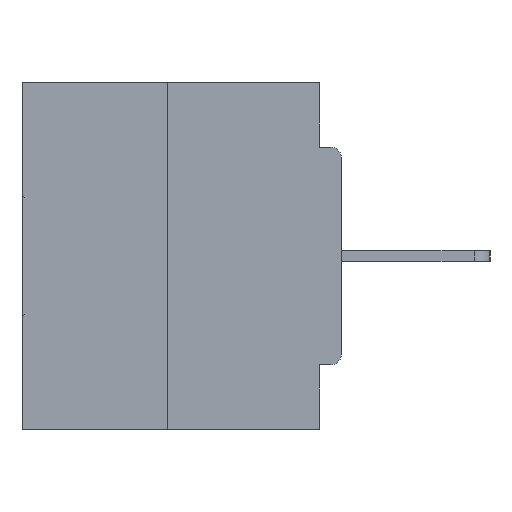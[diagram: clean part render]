
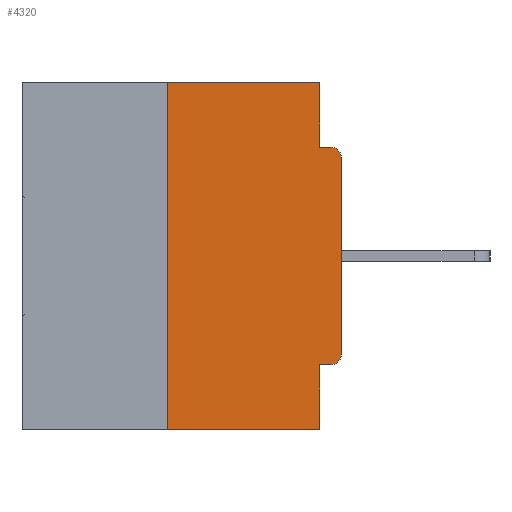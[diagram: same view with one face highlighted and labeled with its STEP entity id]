
A CAD part, left-side view. The second image highlights one B-rep face of the part: STEP entity #4320.
In plain terms, the highlighted planar face has unit normal (-1, 0, 0).
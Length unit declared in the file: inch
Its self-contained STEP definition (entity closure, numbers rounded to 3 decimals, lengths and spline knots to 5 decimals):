
#682 = VERTEX_POINT ( 'NONE', #20227 ) ;
#1584 = LINE ( 'NONE', #30720, #3034 ) ;
#2029 = CARTESIAN_POINT ( 'NONE',  ( 0., 0.46, -0.5 ) ) ;
#2824 = DIRECTION ( 'NONE',  ( 0., 0., -1. ) ) ;
#2882 = CARTESIAN_POINT ( 'NONE',  ( 0., 0.015, -0.3915 ) ) ;
#3034 = VECTOR ( 'NONE', #12272, 39.37008 ) ;
#3341 = AXIS2_PLACEMENT_3D ( 'NONE', #2882, #26212, #32212 ) ;
#3431 = FACE_OUTER_BOUND ( 'NONE', #16127, .T. ) ;
#3579 = CARTESIAN_POINT ( 'NONE',  ( 0., 0.031, -0.5 ) ) ;
#3652 = VECTOR ( 'NONE', #10860, 39.37008 ) ;
#4320 = ADVANCED_FACE ( 'NONE', ( #3431 ), #11691, .F. ) ;
#5598 = ORIENTED_EDGE ( 'NONE', *, *, #26268, .F. ) ;
#5643 = LINE ( 'NONE', #26154, #33511 ) ;
#5899 = ORIENTED_EDGE ( 'NONE', *, *, #22639, .F. ) ;
#5912 = DIRECTION ( 'NONE',  ( 0., 0., -1. ) ) ;
#6058 = CARTESIAN_POINT ( 'NONE',  ( 0., 0.46, 0. ) ) ;
#6705 = DIRECTION ( 'NONE',  ( 0., -1., 0. ) ) ;
#6712 = ORIENTED_EDGE ( 'NONE', *, *, #23414, .T. ) ;
#8031 = VERTEX_POINT ( 'NONE', #10395 ) ;
#8466 = LINE ( 'NONE', #16094, #3652 ) ;
#8569 = EDGE_CURVE ( 'NONE', #27784, #20733, #15224, .T. ) ;
#8991 = EDGE_CURVE ( 'NONE', #27376, #682, #29755, .T. ) ;
#9365 = ORIENTED_EDGE ( 'NONE', *, *, #18132, .F. ) ;
#9810 = VECTOR ( 'NONE', #17044, 39.37008 ) ;
#10395 = CARTESIAN_POINT ( 'NONE',  ( 0., 0.25, -0.5 ) ) ;
#10860 = DIRECTION ( 'NONE',  ( 0., 0., -1. ) ) ;
#11357 = CARTESIAN_POINT ( 'NONE',  ( 0., 0.46, 0. ) ) ;
#11560 = VERTEX_POINT ( 'NONE', #32696 ) ;
#11629 = CARTESIAN_POINT ( 'NONE',  ( 0., 0., 0. ) ) ;
#11691 = PLANE ( 'NONE',  #19172 ) ;
#12044 = CARTESIAN_POINT ( 'NONE',  ( 0., 0.015, -0.1085 ) ) ;
#12272 = DIRECTION ( 'NONE',  ( 0., -1., 0. ) ) ;
#12389 = ORIENTED_EDGE ( 'NONE', *, *, #8991, .T. ) ;
#12974 = VERTEX_POINT ( 'NONE', #33883 ) ;
#13662 = DIRECTION ( 'NONE',  ( 0., 0., 1. ) ) ;
#13952 = CARTESIAN_POINT ( 'NONE',  ( 0., 0.031, -0.0935 ) ) ;
#14004 = CARTESIAN_POINT ( 'NONE',  ( 0., 0.25, 0. ) ) ;
#14113 = AXIS2_PLACEMENT_3D ( 'NONE', #12044, #17453, #5912 ) ;
#14368 = EDGE_CURVE ( 'NONE', #20733, #32277, #15974, .T. ) ;
#15224 = LINE ( 'NONE', #6058, #17228 ) ;
#15974 = LINE ( 'NONE', #26608, #23250 ) ;
#16094 = CARTESIAN_POINT ( 'NONE',  ( 0., 0.031, -0.5 ) ) ;
#16127 = EDGE_LOOP ( 'NONE', ( #33001, #34014, #30296, #5598, #9365, #22301, #12389, #6712, #5899, #24983 ) ) ;
#17044 = DIRECTION ( 'NONE',  ( 0., 0., 1. ) ) ;
#17228 = VECTOR ( 'NONE', #6705, 39.37008 ) ;
#17453 = DIRECTION ( 'NONE',  ( -1., 0., 0. ) ) ;
#17992 = EDGE_CURVE ( 'NONE', #8031, #28303, #20064, .T. ) ;
#18132 = EDGE_CURVE ( 'NONE', #11560, #12974, #5643, .T. ) ;
#18312 = CIRCLE ( 'NONE', #3341, 0.015 ) ;
#18964 = CARTESIAN_POINT ( 'NONE',  ( 0., 0.031, 0. ) ) ;
#19172 = AXIS2_PLACEMENT_3D ( 'NONE', #11357, #19394, #30494 ) ;
#19394 = DIRECTION ( 'NONE',  ( 1., 0., 0. ) ) ;
#20064 = LINE ( 'NONE', #2029, #26854 ) ;
#20227 = CARTESIAN_POINT ( 'NONE',  ( 0., 0., -0.1085 ) ) ;
#20625 = VERTEX_POINT ( 'NONE', #23519 ) ;
#20733 = VERTEX_POINT ( 'NONE', #18964 ) ;
#21195 = EDGE_CURVE ( 'NONE', #8031, #27784, #21532, .T. ) ;
#21532 = LINE ( 'NONE', #14004, #24099 ) ;
#22301 = ORIENTED_EDGE ( 'NONE', *, *, #33808, .T. ) ;
#22639 = EDGE_CURVE ( 'NONE', #32277, #20625, #1584, .T. ) ;
#22945 = CARTESIAN_POINT ( 'NONE',  ( 0., 0., -0.3915 ) ) ;
#23250 = VECTOR ( 'NONE', #2824, 39.37008 ) ;
#23414 = EDGE_CURVE ( 'NONE', #682, #20625, #33563, .T. ) ;
#23519 = CARTESIAN_POINT ( 'NONE',  ( 0., 0.015, -0.0935 ) ) ;
#24034 = DIRECTION ( 'NONE',  ( 0., 1., 0. ) ) ;
#24099 = VECTOR ( 'NONE', #13662, 39.37008 ) ;
#24983 = ORIENTED_EDGE ( 'NONE', *, *, #14368, .F. ) ;
#26154 = CARTESIAN_POINT ( 'NONE',  ( 0., 0., -0.4065 ) ) ;
#26212 = DIRECTION ( 'NONE',  ( -1., 0., 0. ) ) ;
#26268 = EDGE_CURVE ( 'NONE', #12974, #28303, #8466, .T. ) ;
#26608 = CARTESIAN_POINT ( 'NONE',  ( 0., 0.031, 0. ) ) ;
#26854 = VECTOR ( 'NONE', #30831, 39.37008 ) ;
#27376 = VERTEX_POINT ( 'NONE', #22945 ) ;
#27784 = VERTEX_POINT ( 'NONE', #32421 ) ;
#28303 = VERTEX_POINT ( 'NONE', #3579 ) ;
#29755 = LINE ( 'NONE', #11629, #9810 ) ;
#30296 = ORIENTED_EDGE ( 'NONE', *, *, #17992, .T. ) ;
#30494 = DIRECTION ( 'NONE',  ( 0., 0., -1. ) ) ;
#30720 = CARTESIAN_POINT ( 'NONE',  ( 0., 0., -0.0935 ) ) ;
#30831 = DIRECTION ( 'NONE',  ( 0., -1., 0. ) ) ;
#32212 = DIRECTION ( 'NONE',  ( 0., 0., -1. ) ) ;
#32277 = VERTEX_POINT ( 'NONE', #13952 ) ;
#32421 = CARTESIAN_POINT ( 'NONE',  ( 0., 0.25, 0. ) ) ;
#32696 = CARTESIAN_POINT ( 'NONE',  ( 0., 0.015, -0.4065 ) ) ;
#33001 = ORIENTED_EDGE ( 'NONE', *, *, #8569, .F. ) ;
#33511 = VECTOR ( 'NONE', #24034, 39.37008 ) ;
#33563 = CIRCLE ( 'NONE', #14113, 0.015 ) ;
#33808 = EDGE_CURVE ( 'NONE', #11560, #27376, #18312, .T. ) ;
#33883 = CARTESIAN_POINT ( 'NONE',  ( 0., 0.031, -0.4065 ) ) ;
#34014 = ORIENTED_EDGE ( 'NONE', *, *, #21195, .F. ) ;
